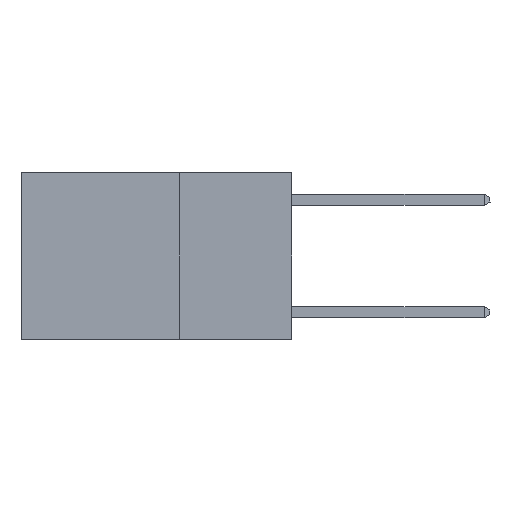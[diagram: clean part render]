
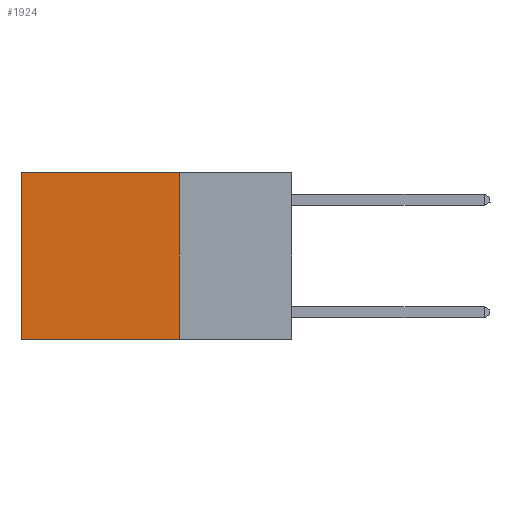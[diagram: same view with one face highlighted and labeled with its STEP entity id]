
A CAD part, left-side view. The second image highlights one B-rep face of the part: STEP entity #1924.
In plain terms, the highlighted planar face has unit normal (-1, 0, 0).
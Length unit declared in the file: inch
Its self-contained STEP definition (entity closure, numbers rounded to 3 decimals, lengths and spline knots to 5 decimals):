
#416 = EDGE_CURVE ( 'NONE', #17089, #5187, #9327, .T. ) ;
#493 = VECTOR ( 'NONE', #20309, 39.37008 ) ;
#1061 = PLANE ( 'NONE',  #17243 ) ;
#1687 = VERTEX_POINT ( 'NONE', #5690 ) ;
#1924 = ADVANCED_FACE ( 'NONE', ( #19281 ), #1061, .F. ) ;
#2628 = CARTESIAN_POINT ( 'NONE',  ( 0.2625, 0.25, -0.37 ) ) ;
#3811 = ORIENTED_EDGE ( 'NONE', *, *, #8015, .F. ) ;
#4182 = LINE ( 'NONE', #17925, #20189 ) ;
#5048 = CARTESIAN_POINT ( 'NONE',  ( 0.2625, 0.6, -0.37 ) ) ;
#5187 = VERTEX_POINT ( 'NONE', #5048 ) ;
#5482 = CARTESIAN_POINT ( 'NONE',  ( 0.2625, 0.6, 0. ) ) ;
#5522 = EDGE_LOOP ( 'NONE', ( #7306, #18188, #3811, #9970 ) ) ;
#5690 = CARTESIAN_POINT ( 'NONE',  ( 0.2625, 0.25, 0. ) ) ;
#5779 = CARTESIAN_POINT ( 'NONE',  ( 0.2625, 0.25, -0.37 ) ) ;
#5782 = VERTEX_POINT ( 'NONE', #5779 ) ;
#7306 = ORIENTED_EDGE ( 'NONE', *, *, #416, .T. ) ;
#8015 = EDGE_CURVE ( 'NONE', #1687, #5782, #20099, .T. ) ;
#9327 = LINE ( 'NONE', #9776, #22326 ) ;
#9649 = DIRECTION ( 'NONE',  ( 0., 0., -1. ) ) ;
#9776 = CARTESIAN_POINT ( 'NONE',  ( 0.2625, 0.6, 0. ) ) ;
#9970 = ORIENTED_EDGE ( 'NONE', *, *, #16233, .T. ) ;
#10416 = DIRECTION ( 'NONE',  ( 0., 0., -1. ) ) ;
#15808 = DIRECTION ( 'NONE',  ( 0., 1., 0. ) ) ;
#16233 = EDGE_CURVE ( 'NONE', #1687, #17089, #4182, .T. ) ;
#16282 = DIRECTION ( 'NONE',  ( 1., 0., 0. ) ) ;
#17089 = VERTEX_POINT ( 'NONE', #5482 ) ;
#17243 = AXIS2_PLACEMENT_3D ( 'NONE', #22029, #16282, #10416 ) ;
#17925 = CARTESIAN_POINT ( 'NONE',  ( 0.2625, 0.25, 0. ) ) ;
#18188 = ORIENTED_EDGE ( 'NONE', *, *, #20017, .F. ) ;
#19281 = FACE_OUTER_BOUND ( 'NONE', #5522, .T. ) ;
#19500 = VECTOR ( 'NONE', #9649, 39.37008 ) ;
#20017 = EDGE_CURVE ( 'NONE', #5782, #5187, #22186, .T. ) ;
#20099 = LINE ( 'NONE', #23306, #19500 ) ;
#20189 = VECTOR ( 'NONE', #15808, 39.37008 ) ;
#20309 = DIRECTION ( 'NONE',  ( 0., 1., 0. ) ) ;
#22029 = CARTESIAN_POINT ( 'NONE',  ( 0.2625, 0.25, 0. ) ) ;
#22186 = LINE ( 'NONE', #2628, #493 ) ;
#22326 = VECTOR ( 'NONE', #23128, 39.37008 ) ;
#23128 = DIRECTION ( 'NONE',  ( 0., 0., -1. ) ) ;
#23306 = CARTESIAN_POINT ( 'NONE',  ( 0.2625, 0.25, 0. ) ) ;
